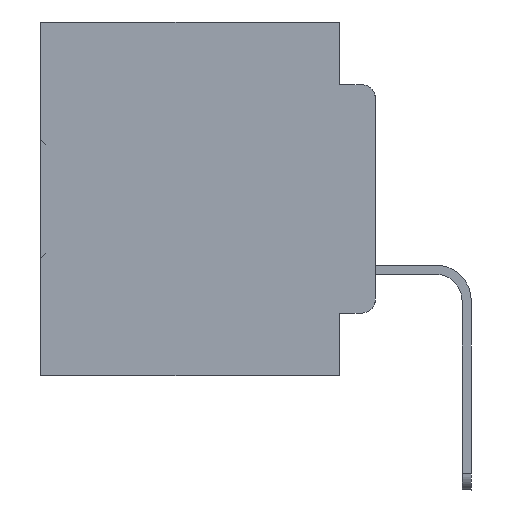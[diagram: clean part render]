
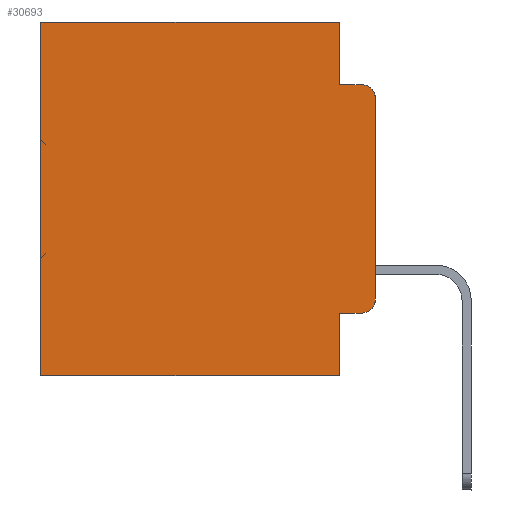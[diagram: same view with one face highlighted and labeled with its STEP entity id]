
A CAD part, left-side view. The second image highlights one B-rep face of the part: STEP entity #30693.
In plain terms, the highlighted planar face has unit normal (-1, 0, 0).
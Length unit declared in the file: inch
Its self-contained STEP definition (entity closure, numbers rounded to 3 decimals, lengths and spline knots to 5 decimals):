
#254 = EDGE_CURVE ( 'NONE', #16882, #4454, #35894, .T. ) ;
#881 = DIRECTION ( 'NONE',  ( -1., 0., 0. ) ) ;
#1074 = CARTESIAN_POINT ( 'NONE',  ( 0.298, 0., 0. ) ) ;
#1100 = ORIENTED_EDGE ( 'NONE', *, *, #35101, .T. ) ;
#2988 = CARTESIAN_POINT ( 'NONE',  ( 0.298, 0.02, -0.0885 ) ) ;
#3547 = ORIENTED_EDGE ( 'NONE', *, *, #36120, .T. ) ;
#4027 = CIRCLE ( 'NONE', #6807, 0.02 ) ;
#4226 = DIRECTION ( 'NONE',  ( 0., 1., 0. ) ) ;
#4431 = CARTESIAN_POINT ( 'NONE',  ( 0.298, 0.051, 0. ) ) ;
#4454 = VERTEX_POINT ( 'NONE', #25600 ) ;
#4709 = ORIENTED_EDGE ( 'NONE', *, *, #9078, .T. ) ;
#5054 = EDGE_CURVE ( 'NONE', #31914, #18447, #35083, .T. ) ;
#5139 = CARTESIAN_POINT ( 'NONE',  ( 0.298, 0.473, 0. ) ) ;
#5713 = DIRECTION ( 'NONE',  ( 0., 0., -1. ) ) ;
#5961 = EDGE_CURVE ( 'NONE', #35380, #30271, #23035, .T. ) ;
#5983 = VECTOR ( 'NONE', #7248, 39.37008 ) ;
#6100 = EDGE_LOOP ( 'NONE', ( #27820, #3547, #10385, #18605, #20329, #4709, #31054, #22880, #8855, #1100 ) ) ;
#6807 = AXIS2_PLACEMENT_3D ( 'NONE', #8436, #34343, #5713 ) ;
#7076 = DIRECTION ( 'NONE',  ( 1., 0., 0. ) ) ;
#7248 = DIRECTION ( 'NONE',  ( 0., 0., -1. ) ) ;
#7430 = LINE ( 'NONE', #28928, #12236 ) ;
#7535 = CARTESIAN_POINT ( 'NONE',  ( 0.298, 0.051, -0.4115 ) ) ;
#8112 = CIRCLE ( 'NONE', #31622, 0.02 ) ;
#8144 = VERTEX_POINT ( 'NONE', #35336 ) ;
#8436 = CARTESIAN_POINT ( 'NONE',  ( 0.298, 0.02, -0.1085 ) ) ;
#8855 = ORIENTED_EDGE ( 'NONE', *, *, #30609, .T. ) ;
#9078 = EDGE_CURVE ( 'NONE', #30271, #18447, #23367, .T. ) ;
#10385 = ORIENTED_EDGE ( 'NONE', *, *, #15375, .F. ) ;
#11460 = VECTOR ( 'NONE', #22748, 39.37008 ) ;
#12236 = VECTOR ( 'NONE', #31896, 39.37008 ) ;
#12547 = CARTESIAN_POINT ( 'NONE',  ( 0.298, 0.473, -0.5 ) ) ;
#12822 = CARTESIAN_POINT ( 'NONE',  ( 0.298, 0., 0. ) ) ;
#12957 = VERTEX_POINT ( 'NONE', #2988 ) ;
#14634 = VECTOR ( 'NONE', #4226, 39.37008 ) ;
#15375 = EDGE_CURVE ( 'NONE', #21487, #12957, #18075, .T. ) ;
#16882 = VERTEX_POINT ( 'NONE', #24886 ) ;
#17233 = CARTESIAN_POINT ( 'NONE',  ( 0.298, 0.02, -0.3915 ) ) ;
#17925 = VECTOR ( 'NONE', #23743, 39.37008 ) ;
#18075 = LINE ( 'NONE', #28229, #11460 ) ;
#18447 = VERTEX_POINT ( 'NONE', #12547 ) ;
#18605 = ORIENTED_EDGE ( 'NONE', *, *, #32895, .F. ) ;
#18936 = CARTESIAN_POINT ( 'NONE',  ( 0.298, 0.051, 0. ) ) ;
#19212 = CARTESIAN_POINT ( 'NONE',  ( 0.298, 0.051, -0.0885 ) ) ;
#20042 = DIRECTION ( 'NONE',  ( 0., 0., -1. ) ) ;
#20329 = ORIENTED_EDGE ( 'NONE', *, *, #5961, .T. ) ;
#20549 = LINE ( 'NONE', #26244, #17925 ) ;
#20571 = CARTESIAN_POINT ( 'NONE',  ( 0.298, 0.051, -0.5 ) ) ;
#20640 = CARTESIAN_POINT ( 'NONE',  ( 0.298, 0.473, 0. ) ) ;
#21487 = VERTEX_POINT ( 'NONE', #19212 ) ;
#22748 = DIRECTION ( 'NONE',  ( 0., -1., 0. ) ) ;
#22880 = ORIENTED_EDGE ( 'NONE', *, *, #32699, .F. ) ;
#23035 = LINE ( 'NONE', #12822, #14634 ) ;
#23367 = LINE ( 'NONE', #20640, #31391 ) ;
#23743 = DIRECTION ( 'NONE',  ( 0., 0., -1. ) ) ;
#24886 = CARTESIAN_POINT ( 'NONE',  ( 0.298, 0., -0.1085 ) ) ;
#25600 = CARTESIAN_POINT ( 'NONE',  ( 0.298, 0., -0.3915 ) ) ;
#26233 = DIRECTION ( 'NONE',  ( 0., 0., -1. ) ) ;
#26244 = CARTESIAN_POINT ( 'NONE',  ( 0.298, 0.051, 0. ) ) ;
#26809 = PLANE ( 'NONE',  #36006 ) ;
#27453 = DIRECTION ( 'NONE',  ( 0., 1., 0. ) ) ;
#27820 = ORIENTED_EDGE ( 'NONE', *, *, #254, .F. ) ;
#28229 = CARTESIAN_POINT ( 'NONE',  ( 0.298, 0.051, -0.0885 ) ) ;
#28928 = CARTESIAN_POINT ( 'NONE',  ( 0.298, 0.051, -0.4115 ) ) ;
#29422 = DIRECTION ( 'NONE',  ( 0., 0., -1. ) ) ;
#29528 = FACE_OUTER_BOUND ( 'NONE', #6100, .T. ) ;
#29674 = CARTESIAN_POINT ( 'NONE',  ( 0.298, 0., 0. ) ) ;
#30271 = VERTEX_POINT ( 'NONE', #5139 ) ;
#30609 = EDGE_CURVE ( 'NONE', #32279, #8144, #7430, .T. ) ;
#30693 = ADVANCED_FACE ( 'NONE', ( #29528 ), #26809, .F. ) ;
#31054 = ORIENTED_EDGE ( 'NONE', *, *, #5054, .F. ) ;
#31391 = VECTOR ( 'NONE', #26233, 39.37008 ) ;
#31622 = AXIS2_PLACEMENT_3D ( 'NONE', #17233, #881, #20042 ) ;
#31896 = DIRECTION ( 'NONE',  ( 0., -1., 0. ) ) ;
#31914 = VERTEX_POINT ( 'NONE', #20571 ) ;
#32279 = VERTEX_POINT ( 'NONE', #7535 ) ;
#32699 = EDGE_CURVE ( 'NONE', #32279, #31914, #20549, .T. ) ;
#32895 = EDGE_CURVE ( 'NONE', #35380, #21487, #33826, .T. ) ;
#33826 = LINE ( 'NONE', #4431, #5983 ) ;
#34343 = DIRECTION ( 'NONE',  ( -1., 0., 0. ) ) ;
#34975 = DIRECTION ( 'NONE',  ( 0., 0., -1. ) ) ;
#35083 = LINE ( 'NONE', #36458, #36417 ) ;
#35101 = EDGE_CURVE ( 'NONE', #8144, #4454, #8112, .T. ) ;
#35336 = CARTESIAN_POINT ( 'NONE',  ( 0.298, 0.02, -0.4115 ) ) ;
#35380 = VERTEX_POINT ( 'NONE', #18936 ) ;
#35482 = VECTOR ( 'NONE', #29422, 39.37008 ) ;
#35894 = LINE ( 'NONE', #1074, #35482 ) ;
#36006 = AXIS2_PLACEMENT_3D ( 'NONE', #29674, #7076, #34975 ) ;
#36120 = EDGE_CURVE ( 'NONE', #16882, #12957, #4027, .T. ) ;
#36417 = VECTOR ( 'NONE', #27453, 39.37008 ) ;
#36458 = CARTESIAN_POINT ( 'NONE',  ( 0.298, 0., -0.5 ) ) ;
